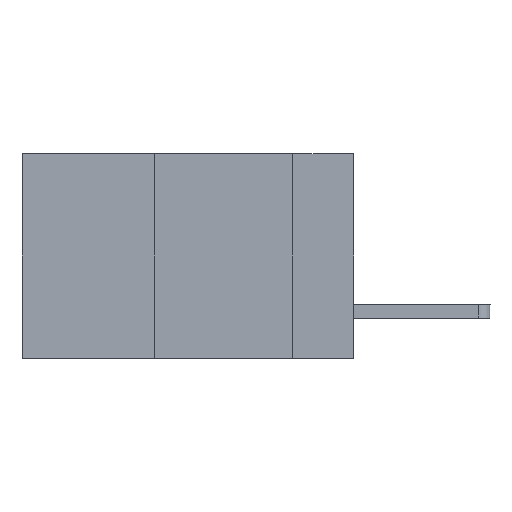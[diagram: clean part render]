
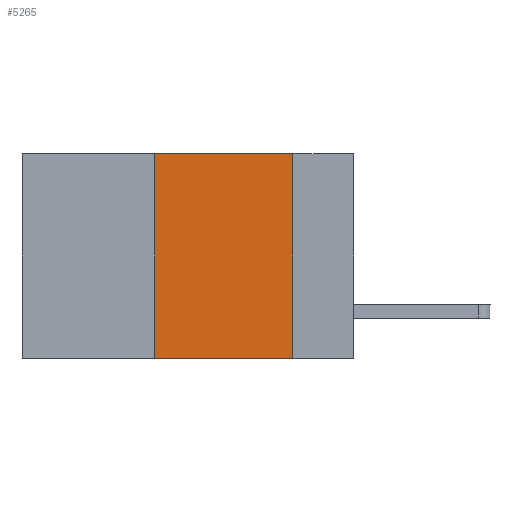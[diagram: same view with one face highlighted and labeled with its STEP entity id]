
A CAD part, left-side view. The second image highlights one B-rep face of the part: STEP entity #5265.
In plain terms, the highlighted planar face has unit normal (-1, 0, 0).
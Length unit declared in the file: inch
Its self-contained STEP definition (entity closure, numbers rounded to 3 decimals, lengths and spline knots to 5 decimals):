
#67 = ORIENTED_EDGE ( 'NONE', *, *, #8096, .F. ) ;
#235 = ORIENTED_EDGE ( 'NONE', *, *, #3382, .T. ) ;
#291 = LINE ( 'NONE', #8709, #8591 ) ;
#310 = PLANE ( 'NONE',  #975 ) ;
#361 = DIRECTION ( 'NONE',  ( 0., 0., 1. ) ) ;
#481 = CARTESIAN_POINT ( 'NONE',  ( 0., 0.11, 0. ) ) ;
#975 = AXIS2_PLACEMENT_3D ( 'NONE', #5049, #2339, #985 ) ;
#985 = DIRECTION ( 'NONE',  ( 0., 0., -1. ) ) ;
#1043 = VECTOR ( 'NONE', #6230, 39.37008 ) ;
#1053 = CARTESIAN_POINT ( 'NONE',  ( 0., 0.36, 0. ) ) ;
#1392 = CARTESIAN_POINT ( 'NONE',  ( 0., 0.6, -0.37 ) ) ;
#1633 = CARTESIAN_POINT ( 'NONE',  ( 0., 0.36, 0. ) ) ;
#1863 = VECTOR ( 'NONE', #361, 39.37008 ) ;
#1868 = EDGE_LOOP ( 'NONE', ( #6798, #4450, #67, #235 ) ) ;
#2075 = VERTEX_POINT ( 'NONE', #7972 ) ;
#2145 = VERTEX_POINT ( 'NONE', #6173 ) ;
#2295 = EDGE_CURVE ( 'NONE', #7238, #8247, #3391, .T. ) ;
#2339 = DIRECTION ( 'NONE',  ( 1., 0., 0. ) ) ;
#3256 = DIRECTION ( 'NONE',  ( 0., 0., -1. ) ) ;
#3382 = EDGE_CURVE ( 'NONE', #2145, #2075, #6939, .T. ) ;
#3391 = LINE ( 'NONE', #6345, #1043 ) ;
#3671 = LINE ( 'NONE', #1633, #1863 ) ;
#4450 = ORIENTED_EDGE ( 'NONE', *, *, #2295, .F. ) ;
#5049 = CARTESIAN_POINT ( 'NONE',  ( 0., 0.6, 0. ) ) ;
#5265 = ADVANCED_FACE ( 'NONE', ( #6275 ), #310, .F. ) ;
#6173 = CARTESIAN_POINT ( 'NONE',  ( 0., 0.36, -0.37 ) ) ;
#6230 = DIRECTION ( 'NONE',  ( 0., -1., 0. ) ) ;
#6275 = FACE_OUTER_BOUND ( 'NONE', #1868, .T. ) ;
#6345 = CARTESIAN_POINT ( 'NONE',  ( 0., 0.6, 0. ) ) ;
#6798 = ORIENTED_EDGE ( 'NONE', *, *, #7554, .F. ) ;
#6939 = LINE ( 'NONE', #1392, #7356 ) ;
#7238 = VERTEX_POINT ( 'NONE', #1053 ) ;
#7356 = VECTOR ( 'NONE', #8234, 39.37008 ) ;
#7554 = EDGE_CURVE ( 'NONE', #8247, #2075, #291, .T. ) ;
#7972 = CARTESIAN_POINT ( 'NONE',  ( 0., 0.11, -0.37 ) ) ;
#8096 = EDGE_CURVE ( 'NONE', #2145, #7238, #3671, .T. ) ;
#8234 = DIRECTION ( 'NONE',  ( 0., -1., 0. ) ) ;
#8247 = VERTEX_POINT ( 'NONE', #481 ) ;
#8591 = VECTOR ( 'NONE', #3256, 39.37008 ) ;
#8709 = CARTESIAN_POINT ( 'NONE',  ( 0., 0.11, 0. ) ) ;
